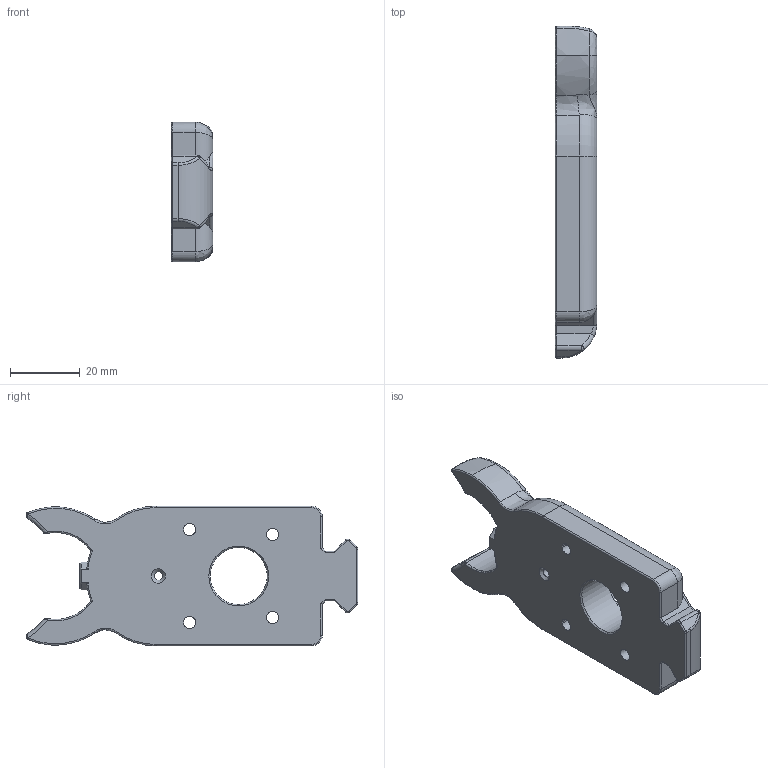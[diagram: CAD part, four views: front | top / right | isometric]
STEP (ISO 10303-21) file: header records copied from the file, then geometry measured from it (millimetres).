
FILE_DESCRIPTION (( 'STEP AP203' ), '1' );
FILE_NAME ('WTF-9_barrel_retainer_cap.STEP', '2020-05-09T09:28:44', ( '' ), ( '' ), 'SwSTEP 2.0', 'SolidWorks 2016', '' );
FILE_SCHEMA (( 'CONFIG_CONTROL_DESIGN' ));
Length unit declared in the file: millimetre
Products named in the file (2): WTF9 V1 FINAL_17; WTF-9_barrel_retainer_cap
Assembly tree (1 placements, depth 2):
  WTF-9_barrel_retainer_cap
    WTF9 V1 FINAL_17
Bounding box: 12 x 95.49 x 40.2 mm (x, y, z)
Volume: 31800.5 mm3; surface area: 9857.7 mm2
Topology: 1 solids, 1 shells, 139 faces, 349 edges, 205 vertices
Faces by surface type: cylinder 42, bspline 36, plane 34, torus 23, cone 2, sphere 2
Full cylindrical faces by diameter (mm): 2.5 x2, 3.5 x2, 16.4 x1
Entity records: 6127 total; most frequent: CARTESIAN_POINT 3043, ORIENTED_EDGE 670, DIRECTION 487, EDGE_CURVE 335, VERTEX_POINT 205, AXIS2_PLACEMENT_3D 188, EDGE_LOOP 158, FACE_OUTER_BOUND 145
